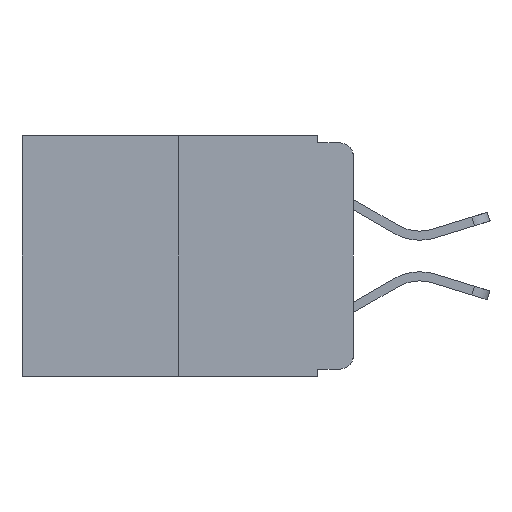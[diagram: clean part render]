
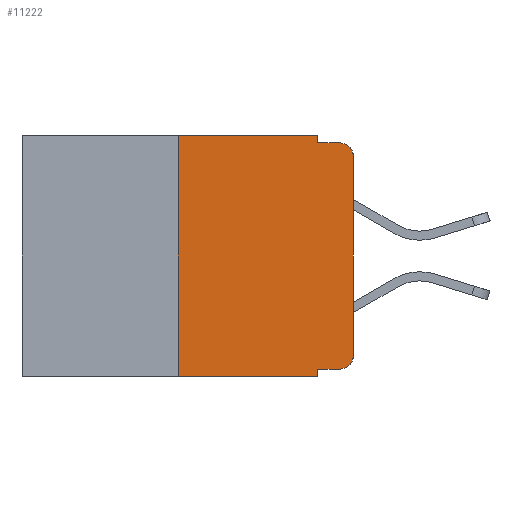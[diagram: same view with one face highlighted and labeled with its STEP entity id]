
A CAD part, left-side view. The second image highlights one B-rep face of the part: STEP entity #11222.
In plain terms, the highlighted planar face has unit normal (-1, 0, 0).
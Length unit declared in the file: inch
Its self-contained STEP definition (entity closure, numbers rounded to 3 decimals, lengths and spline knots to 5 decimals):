
#180 = CARTESIAN_POINT ( 'NONE',  ( 0., 0.473, 0. ) ) ;
#613 = VERTEX_POINT ( 'NONE', #11454 ) ;
#703 = ORIENTED_EDGE ( 'NONE', *, *, #3083, .F. ) ;
#772 = AXIS2_PLACEMENT_3D ( 'NONE', #6893, #13961, #7975 ) ;
#974 = CARTESIAN_POINT ( 'NONE',  ( 0., 0.051, -0.01 ) ) ;
#1288 = ORIENTED_EDGE ( 'NONE', *, *, #9618, .T. ) ;
#1307 = DIRECTION ( 'NONE',  ( -1., 0., 0. ) ) ;
#1700 = CIRCLE ( 'NONE', #5796, 0.02 ) ;
#2047 = CARTESIAN_POINT ( 'NONE',  ( 0., 0.051, 0. ) ) ;
#2339 = LINE ( 'NONE', #8430, #7591 ) ;
#2480 = CARTESIAN_POINT ( 'NONE',  ( 0., 0.051, 0. ) ) ;
#2718 = LINE ( 'NONE', #7102, #3081 ) ;
#2996 = EDGE_CURVE ( 'NONE', #613, #4318, #2339, .T. ) ;
#3081 = VECTOR ( 'NONE', #8166, 39.37008 ) ;
#3083 = EDGE_CURVE ( 'NONE', #12893, #4539, #9674, .T. ) ;
#3279 = VERTEX_POINT ( 'NONE', #6114 ) ;
#3728 = VECTOR ( 'NONE', #9031, 39.37008 ) ;
#3766 = EDGE_LOOP ( 'NONE', ( #9310, #12030, #703, #6854, #9769, #4276, #1288, #4424, #12750, #9619 ) ) ;
#3900 = PLANE ( 'NONE',  #7700 ) ;
#4249 = VERTEX_POINT ( 'NONE', #11020 ) ;
#4276 = ORIENTED_EDGE ( 'NONE', *, *, #6833, .F. ) ;
#4318 = VERTEX_POINT ( 'NONE', #2047 ) ;
#4424 = ORIENTED_EDGE ( 'NONE', *, *, #5795, .F. ) ;
#4472 = VECTOR ( 'NONE', #12937, 39.37008 ) ;
#4539 = VERTEX_POINT ( 'NONE', #8055 ) ;
#4639 = CARTESIAN_POINT ( 'NONE',  ( 0., 0., 0. ) ) ;
#4640 = FACE_OUTER_BOUND ( 'NONE', #3766, .T. ) ;
#4667 = VERTEX_POINT ( 'NONE', #7214 ) ;
#4826 = LINE ( 'NONE', #4639, #4472 ) ;
#5023 = DIRECTION ( 'NONE',  ( 1., 0., 0. ) ) ;
#5430 = CARTESIAN_POINT ( 'NONE',  ( 0., 0.02, -0.333 ) ) ;
#5795 = EDGE_CURVE ( 'NONE', #4667, #3279, #9456, .T. ) ;
#5796 = AXIS2_PLACEMENT_3D ( 'NONE', #8071, #1307, #9091 ) ;
#6114 = CARTESIAN_POINT ( 'NONE',  ( 0., 0.051, -0.343 ) ) ;
#6710 = CARTESIAN_POINT ( 'NONE',  ( 0., 0.25, 0. ) ) ;
#6814 = EDGE_CURVE ( 'NONE', #4318, #12893, #9104, .T. ) ;
#6833 = EDGE_CURVE ( 'NONE', #13047, #613, #13791, .T. ) ;
#6854 = ORIENTED_EDGE ( 'NONE', *, *, #6814, .F. ) ;
#6893 = CARTESIAN_POINT ( 'NONE',  ( 0., 0.02, -0.313 ) ) ;
#7063 = CIRCLE ( 'NONE', #772, 0.02 ) ;
#7102 = CARTESIAN_POINT ( 'NONE',  ( 0., 0.473, -0.343 ) ) ;
#7214 = CARTESIAN_POINT ( 'NONE',  ( 0., 0.051, -0.333 ) ) ;
#7436 = VERTEX_POINT ( 'NONE', #5430 ) ;
#7591 = VECTOR ( 'NONE', #8140, 39.37008 ) ;
#7700 = AXIS2_PLACEMENT_3D ( 'NONE', #180, #5023, #12316 ) ;
#7815 = DIRECTION ( 'NONE',  ( 0., 0., 1. ) ) ;
#7975 = DIRECTION ( 'NONE',  ( 0., 0., -1. ) ) ;
#7998 = EDGE_CURVE ( 'NONE', #4667, #7436, #11502, .T. ) ;
#8055 = CARTESIAN_POINT ( 'NONE',  ( 0., 0.02, -0.01 ) ) ;
#8071 = CARTESIAN_POINT ( 'NONE',  ( 0., 0.02, -0.03 ) ) ;
#8140 = DIRECTION ( 'NONE',  ( 0., -1., 0. ) ) ;
#8166 = DIRECTION ( 'NONE',  ( 0., -1., 0. ) ) ;
#8430 = CARTESIAN_POINT ( 'NONE',  ( 0., 0.473, 0. ) ) ;
#8512 = CARTESIAN_POINT ( 'NONE',  ( 0., 0.051, -0.333 ) ) ;
#8753 = VECTOR ( 'NONE', #13498, 39.37008 ) ;
#8795 = DIRECTION ( 'NONE',  ( 0., 0., -1. ) ) ;
#9031 = DIRECTION ( 'NONE',  ( 0., 0., -1. ) ) ;
#9091 = DIRECTION ( 'NONE',  ( 0., 0., -1. ) ) ;
#9104 = LINE ( 'NONE', #13771, #11218 ) ;
#9310 = ORIENTED_EDGE ( 'NONE', *, *, #10942, .T. ) ;
#9456 = LINE ( 'NONE', #2480, #3728 ) ;
#9618 = EDGE_CURVE ( 'NONE', #13047, #3279, #2718, .T. ) ;
#9619 = ORIENTED_EDGE ( 'NONE', *, *, #10992, .T. ) ;
#9674 = LINE ( 'NONE', #974, #11771 ) ;
#9769 = ORIENTED_EDGE ( 'NONE', *, *, #2996, .F. ) ;
#9791 = CARTESIAN_POINT ( 'NONE',  ( 0., 0.051, -0.01 ) ) ;
#10517 = DIRECTION ( 'NONE',  ( 0., -1., 0. ) ) ;
#10903 = VECTOR ( 'NONE', #7815, 39.37008 ) ;
#10942 = EDGE_CURVE ( 'NONE', #12326, #4249, #4826, .T. ) ;
#10992 = EDGE_CURVE ( 'NONE', #7436, #12326, #7063, .T. ) ;
#11014 = CARTESIAN_POINT ( 'NONE',  ( 0., 0.25, -0.343 ) ) ;
#11020 = CARTESIAN_POINT ( 'NONE',  ( 0., 0., -0.03 ) ) ;
#11218 = VECTOR ( 'NONE', #8795, 39.37008 ) ;
#11222 = ADVANCED_FACE ( 'NONE', ( #4640 ), #3900, .F. ) ;
#11454 = CARTESIAN_POINT ( 'NONE',  ( 0., 0.25, 0. ) ) ;
#11502 = LINE ( 'NONE', #8512, #8753 ) ;
#11771 = VECTOR ( 'NONE', #10517, 39.37008 ) ;
#12030 = ORIENTED_EDGE ( 'NONE', *, *, #14022, .T. ) ;
#12316 = DIRECTION ( 'NONE',  ( 0., 0., -1. ) ) ;
#12326 = VERTEX_POINT ( 'NONE', #13808 ) ;
#12750 = ORIENTED_EDGE ( 'NONE', *, *, #7998, .T. ) ;
#12893 = VERTEX_POINT ( 'NONE', #9791 ) ;
#12937 = DIRECTION ( 'NONE',  ( 0., 0., 1. ) ) ;
#13047 = VERTEX_POINT ( 'NONE', #11014 ) ;
#13498 = DIRECTION ( 'NONE',  ( 0., -1., 0. ) ) ;
#13771 = CARTESIAN_POINT ( 'NONE',  ( 0., 0.051, 0. ) ) ;
#13791 = LINE ( 'NONE', #6710, #10903 ) ;
#13808 = CARTESIAN_POINT ( 'NONE',  ( 0., 0., -0.313 ) ) ;
#13961 = DIRECTION ( 'NONE',  ( -1., 0., 0. ) ) ;
#14022 = EDGE_CURVE ( 'NONE', #4249, #4539, #1700, .T. ) ;
